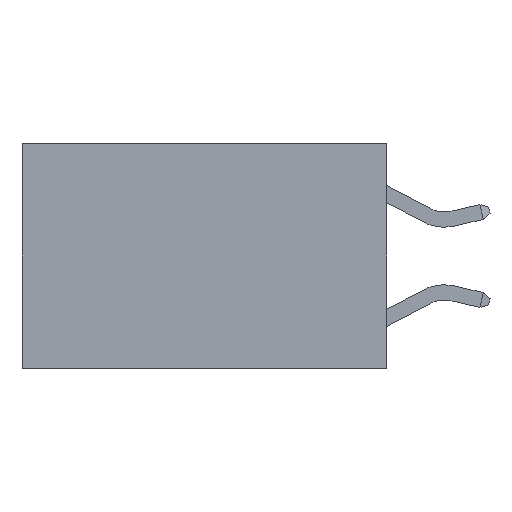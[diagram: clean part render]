
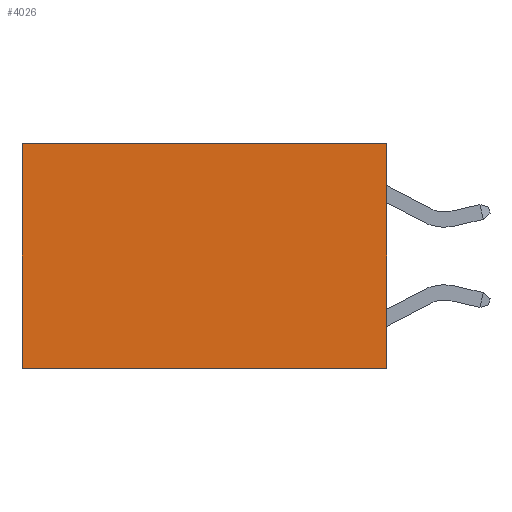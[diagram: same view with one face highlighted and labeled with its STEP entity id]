
A CAD part, left-side view. The second image highlights one B-rep face of the part: STEP entity #4026.
In plain terms, the highlighted planar face has unit normal (-1, 0, 0).
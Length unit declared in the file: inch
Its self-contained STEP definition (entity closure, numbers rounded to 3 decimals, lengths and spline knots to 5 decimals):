
#16 = VECTOR ( 'NONE', #10982, 39.37008 ) ;
#370 = CARTESIAN_POINT ( 'NONE',  ( 0.2625, 0.6, 0. ) ) ;
#534 = EDGE_LOOP ( 'NONE', ( #1796, #10406, #8663, #8413 ) ) ;
#1141 = CARTESIAN_POINT ( 'NONE',  ( 0.2625, 0., 0. ) ) ;
#1796 = ORIENTED_EDGE ( 'NONE', *, *, #3864, .T. ) ;
#2028 = LINE ( 'NONE', #11912, #16 ) ;
#2101 = EDGE_CURVE ( 'NONE', #7828, #7277, #11228, .T. ) ;
#2247 = DIRECTION ( 'NONE',  ( 0., 1., 0. ) ) ;
#3164 = EDGE_CURVE ( 'NONE', #7277, #10796, #12217, .T. ) ;
#3658 = CARTESIAN_POINT ( 'NONE',  ( 0.2625, 0., -0.37 ) ) ;
#3856 = PLANE ( 'NONE',  #4270 ) ;
#3864 = EDGE_CURVE ( 'NONE', #4244, #10796, #4602, .T. ) ;
#4026 = ADVANCED_FACE ( 'NONE', ( #6786 ), #3856, .F. ) ;
#4204 = CARTESIAN_POINT ( 'NONE',  ( 0.2625, 0.6, -0.37 ) ) ;
#4244 = VERTEX_POINT ( 'NONE', #370 ) ;
#4270 = AXIS2_PLACEMENT_3D ( 'NONE', #1141, #7860, #11202 ) ;
#4602 = LINE ( 'NONE', #11619, #11487 ) ;
#5184 = CARTESIAN_POINT ( 'NONE',  ( 0.2625, 0., 0. ) ) ;
#5338 = EDGE_CURVE ( 'NONE', #7828, #4244, #2028, .T. ) ;
#6701 = CARTESIAN_POINT ( 'NONE',  ( 0.2625, 0., 0. ) ) ;
#6786 = FACE_OUTER_BOUND ( 'NONE', #534, .T. ) ;
#7277 = VERTEX_POINT ( 'NONE', #3658 ) ;
#7828 = VERTEX_POINT ( 'NONE', #5184 ) ;
#7860 = DIRECTION ( 'NONE',  ( 1., 0., 0. ) ) ;
#8413 = ORIENTED_EDGE ( 'NONE', *, *, #5338, .T. ) ;
#8473 = DIRECTION ( 'NONE',  ( 0., 0., -1. ) ) ;
#8544 = VECTOR ( 'NONE', #8473, 39.37008 ) ;
#8663 = ORIENTED_EDGE ( 'NONE', *, *, #2101, .F. ) ;
#9466 = DIRECTION ( 'NONE',  ( 0., 0., -1. ) ) ;
#10406 = ORIENTED_EDGE ( 'NONE', *, *, #3164, .F. ) ;
#10796 = VERTEX_POINT ( 'NONE', #4204 ) ;
#10982 = DIRECTION ( 'NONE',  ( 0., 1., 0. ) ) ;
#11202 = DIRECTION ( 'NONE',  ( 0., 0., -1. ) ) ;
#11228 = LINE ( 'NONE', #6701, #8544 ) ;
#11487 = VECTOR ( 'NONE', #9466, 39.37008 ) ;
#11619 = CARTESIAN_POINT ( 'NONE',  ( 0.2625, 0.6, 0. ) ) ;
#11912 = CARTESIAN_POINT ( 'NONE',  ( 0.2625, 0., 0. ) ) ;
#11929 = VECTOR ( 'NONE', #2247, 39.37008 ) ;
#11968 = CARTESIAN_POINT ( 'NONE',  ( 0.2625, 0., -0.37 ) ) ;
#12217 = LINE ( 'NONE', #11968, #11929 ) ;
